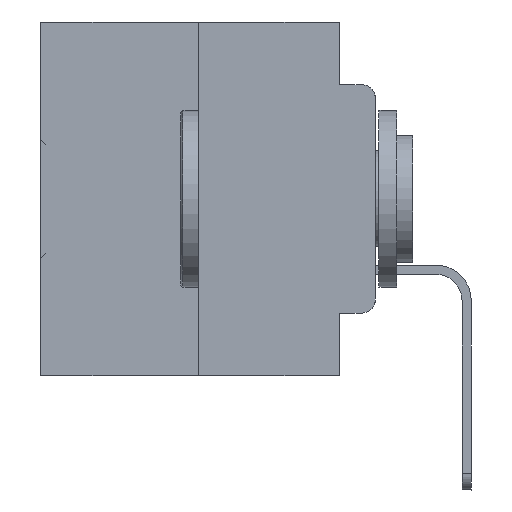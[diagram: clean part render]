
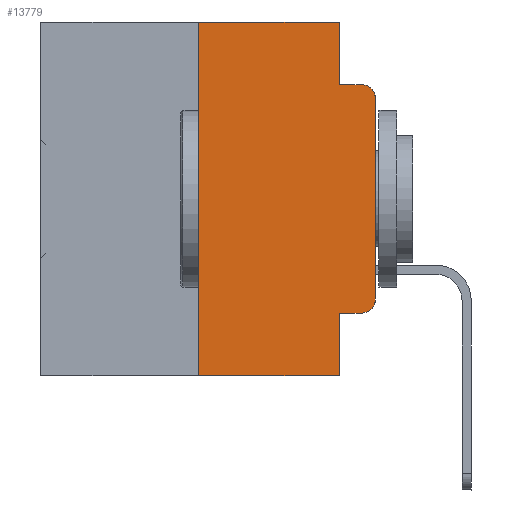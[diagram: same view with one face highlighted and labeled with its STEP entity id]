
A CAD part, left-side view. The second image highlights one B-rep face of the part: STEP entity #13779.
In plain terms, the highlighted planar face has unit normal (-1, 0, 0).
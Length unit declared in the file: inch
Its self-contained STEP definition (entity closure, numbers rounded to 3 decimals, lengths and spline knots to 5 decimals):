
#362 = ORIENTED_EDGE ( 'NONE', *, *, #686, .T. ) ;
#686 = EDGE_CURVE ( 'NONE', #32748, #18008, #19288, .T. ) ;
#772 = DIRECTION ( 'NONE',  ( -1., 0., 0. ) ) ;
#1487 = VECTOR ( 'NONE', #22972, 39.37008 ) ;
#1721 = LINE ( 'NONE', #11881, #12681 ) ;
#2371 = ORIENTED_EDGE ( 'NONE', *, *, #7384, .F. ) ;
#2425 = VERTEX_POINT ( 'NONE', #32688 ) ;
#2806 = VECTOR ( 'NONE', #12311, 39.37008 ) ;
#3439 = ORIENTED_EDGE ( 'NONE', *, *, #4754, .T. ) ;
#3540 = CARTESIAN_POINT ( 'NONE',  ( 0., 0.25, -0.5 ) ) ;
#3655 = CARTESIAN_POINT ( 'NONE',  ( 0., 0.051, 0. ) ) ;
#4167 = CARTESIAN_POINT ( 'NONE',  ( 0., 0.473, 0. ) ) ;
#4666 = FACE_OUTER_BOUND ( 'NONE', #25065, .T. ) ;
#4754 = EDGE_CURVE ( 'NONE', #2425, #22215, #8897, .T. ) ;
#4846 = EDGE_CURVE ( 'NONE', #32565, #31417, #1721, .T. ) ;
#5397 = VECTOR ( 'NONE', #13905, 39.37008 ) ;
#5568 = ORIENTED_EDGE ( 'NONE', *, *, #25936, .F. ) ;
#5722 = CARTESIAN_POINT ( 'NONE',  ( 0., 0.051, -0.4115 ) ) ;
#5779 = CARTESIAN_POINT ( 'NONE',  ( 0., 0.02, -0.3915 ) ) ;
#6235 = DIRECTION ( 'NONE',  ( 0., 0., -1. ) ) ;
#6610 = DIRECTION ( 'NONE',  ( 0., 0., -1. ) ) ;
#6614 = CARTESIAN_POINT ( 'NONE',  ( 0., 0.02, -0.0885 ) ) ;
#6879 = DIRECTION ( 'NONE',  ( 0., 0., -1. ) ) ;
#7384 = EDGE_CURVE ( 'NONE', #31417, #22215, #21334, .T. ) ;
#7425 = VECTOR ( 'NONE', #16987, 39.37008 ) ;
#8897 = CIRCLE ( 'NONE', #17548, 0.02 ) ;
#8981 = CARTESIAN_POINT ( 'NONE',  ( 0., 0.051, -0.0885 ) ) ;
#9070 = VECTOR ( 'NONE', #29737, 39.37008 ) ;
#9988 = CARTESIAN_POINT ( 'NONE',  ( 0., 0., -0.3915 ) ) ;
#10774 = LINE ( 'NONE', #19696, #7425 ) ;
#11198 = CARTESIAN_POINT ( 'NONE',  ( 0., 0.473, -0.5 ) ) ;
#11761 = AXIS2_PLACEMENT_3D ( 'NONE', #4167, #23009, #6879 ) ;
#11881 = CARTESIAN_POINT ( 'NONE',  ( 0., 0.051, 0. ) ) ;
#12311 = DIRECTION ( 'NONE',  ( 0., 0., 1. ) ) ;
#12681 = VECTOR ( 'NONE', #6235, 39.37008 ) ;
#12695 = CARTESIAN_POINT ( 'NONE',  ( 0., 0.051, -0.5 ) ) ;
#13004 = ORIENTED_EDGE ( 'NONE', *, *, #27815, .T. ) ;
#13511 = CARTESIAN_POINT ( 'NONE',  ( 0., 0.051, -0.0885 ) ) ;
#13779 = ADVANCED_FACE ( 'NONE', ( #4666 ), #14884, .F. ) ;
#13795 = ORIENTED_EDGE ( 'NONE', *, *, #16969, .F. ) ;
#13905 = DIRECTION ( 'NONE',  ( 0., -1., 0. ) ) ;
#14884 = PLANE ( 'NONE',  #11761 ) ;
#15422 = LINE ( 'NONE', #20233, #1487 ) ;
#15905 = VERTEX_POINT ( 'NONE', #9988 ) ;
#16705 = CARTESIAN_POINT ( 'NONE',  ( 0., 0.051, -0.4115 ) ) ;
#16969 = EDGE_CURVE ( 'NONE', #32748, #31870, #10774, .T. ) ;
#16987 = DIRECTION ( 'NONE',  ( 0., 0., 1. ) ) ;
#17109 = LINE ( 'NONE', #3655, #30155 ) ;
#17392 = ORIENTED_EDGE ( 'NONE', *, *, #25925, .F. ) ;
#17548 = AXIS2_PLACEMENT_3D ( 'NONE', #25550, #772, #19617 ) ;
#18008 = VERTEX_POINT ( 'NONE', #12695 ) ;
#18070 = VERTEX_POINT ( 'NONE', #20670 ) ;
#18796 = LINE ( 'NONE', #20500, #2806 ) ;
#18935 = CARTESIAN_POINT ( 'NONE',  ( 0., 0.051, 0. ) ) ;
#19288 = LINE ( 'NONE', #11198, #5397 ) ;
#19341 = DIRECTION ( 'NONE',  ( 0., 0., -1. ) ) ;
#19617 = DIRECTION ( 'NONE',  ( 0., 0., -1. ) ) ;
#19696 = CARTESIAN_POINT ( 'NONE',  ( 0., 0.25, 0. ) ) ;
#20233 = CARTESIAN_POINT ( 'NONE',  ( 0., 0.473, 0. ) ) ;
#20500 = CARTESIAN_POINT ( 'NONE',  ( 0., 0., 0. ) ) ;
#20670 = CARTESIAN_POINT ( 'NONE',  ( 0., 0.02, -0.4115 ) ) ;
#21328 = ORIENTED_EDGE ( 'NONE', *, *, #4846, .F. ) ;
#21334 = LINE ( 'NONE', #13511, #30218 ) ;
#22215 = VERTEX_POINT ( 'NONE', #6614 ) ;
#22972 = DIRECTION ( 'NONE',  ( 0., -1., 0. ) ) ;
#23009 = DIRECTION ( 'NONE',  ( 1., 0., 0. ) ) ;
#23340 = DIRECTION ( 'NONE',  ( -1., 0., 0. ) ) ;
#24119 = DIRECTION ( 'NONE',  ( 0., -1., 0. ) ) ;
#24494 = EDGE_CURVE ( 'NONE', #15905, #2425, #18796, .T. ) ;
#25065 = EDGE_LOOP ( 'NONE', ( #28445, #3439, #2371, #21328, #5568, #13795, #362, #17392, #13004, #26800 ) ) ;
#25297 = AXIS2_PLACEMENT_3D ( 'NONE', #5779, #23340, #19341 ) ;
#25550 = CARTESIAN_POINT ( 'NONE',  ( 0., 0.02, -0.1085 ) ) ;
#25925 = EDGE_CURVE ( 'NONE', #28153, #18008, #17109, .T. ) ;
#25936 = EDGE_CURVE ( 'NONE', #31870, #32565, #15422, .T. ) ;
#26497 = EDGE_CURVE ( 'NONE', #18070, #15905, #27587, .T. ) ;
#26800 = ORIENTED_EDGE ( 'NONE', *, *, #26497, .T. ) ;
#27587 = CIRCLE ( 'NONE', #25297, 0.02 ) ;
#27815 = EDGE_CURVE ( 'NONE', #28153, #18070, #29697, .T. ) ;
#28153 = VERTEX_POINT ( 'NONE', #16705 ) ;
#28445 = ORIENTED_EDGE ( 'NONE', *, *, #24494, .T. ) ;
#29697 = LINE ( 'NONE', #5722, #9070 ) ;
#29737 = DIRECTION ( 'NONE',  ( 0., -1., 0. ) ) ;
#30155 = VECTOR ( 'NONE', #6610, 39.37008 ) ;
#30218 = VECTOR ( 'NONE', #24119, 39.37008 ) ;
#31417 = VERTEX_POINT ( 'NONE', #8981 ) ;
#31870 = VERTEX_POINT ( 'NONE', #32255 ) ;
#32255 = CARTESIAN_POINT ( 'NONE',  ( 0., 0.25, 0. ) ) ;
#32565 = VERTEX_POINT ( 'NONE', #18935 ) ;
#32688 = CARTESIAN_POINT ( 'NONE',  ( 0., 0., -0.1085 ) ) ;
#32748 = VERTEX_POINT ( 'NONE', #3540 ) ;
